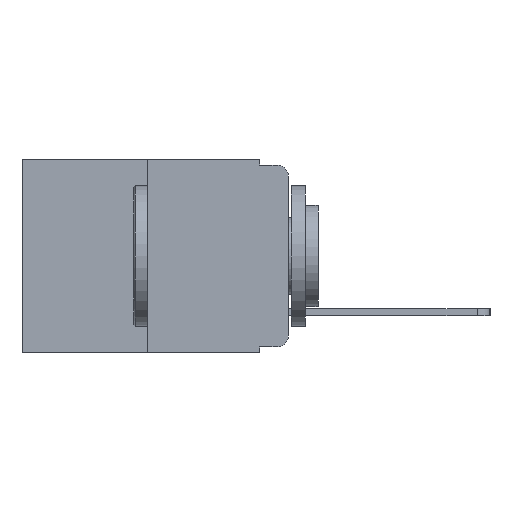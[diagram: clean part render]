
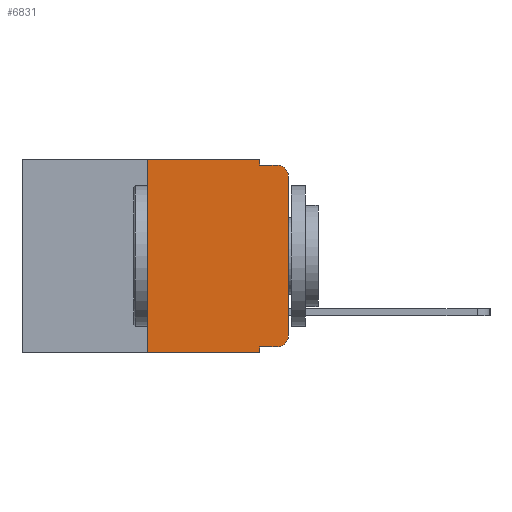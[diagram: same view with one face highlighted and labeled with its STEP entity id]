
A CAD part, left-side view. The second image highlights one B-rep face of the part: STEP entity #6831.
In plain terms, the highlighted planar face has unit normal (-1, 0, 0).
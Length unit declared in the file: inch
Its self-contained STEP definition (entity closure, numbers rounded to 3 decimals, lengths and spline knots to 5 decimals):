
#85 = EDGE_CURVE ( 'NONE', #959, #15943, #3698, .T. ) ;
#376 = EDGE_CURVE ( 'NONE', #1472, #6557, #10152, .T. ) ;
#380 = EDGE_CURVE ( 'NONE', #6557, #20384, #722, .T. ) ;
#412 = EDGE_CURVE ( 'NONE', #9446, #20384, #13553, .T. ) ;
#414 = EDGE_CURVE ( 'NONE', #8505, #9446, #9124, .T. ) ;
#418 = EDGE_CURVE ( 'NONE', #959, #8233, #17444, .T. ) ;
#449 = EDGE_CURVE ( 'NONE', #7345, #15943, #2830, .T. ) ;
#456 = EDGE_CURVE ( 'NONE', #7345, #13118, #6999, .T. ) ;
#485 = EDGE_CURVE ( 'NONE', #13118, #1472, #1667, .T. ) ;
#707 = ORIENTED_EDGE ( 'NONE', *, *, #85, .T. ) ;
#722 = CIRCLE ( 'NONE', #8372, 0.02 ) ;
#959 = VERTEX_POINT ( 'NONE', #21554 ) ;
#1197 = DIRECTION ( 'NONE',  ( 0., -1., 0. ) ) ;
#1244 = DIRECTION ( 'NONE',  ( 0., -1., 0. ) ) ;
#1324 = ORIENTED_EDGE ( 'NONE', *, *, #380, .T. ) ;
#1472 = VERTEX_POINT ( 'NONE', #10882 ) ;
#1580 = CARTESIAN_POINT ( 'NONE',  ( 0., 0.02, -0.313 ) ) ;
#1667 = CIRCLE ( 'NONE', #4444, 0.02 ) ;
#1971 = ORIENTED_EDGE ( 'NONE', *, *, #456, .T. ) ;
#2003 = DIRECTION ( 'NONE',  ( -1., 0., 0. ) ) ;
#2273 = VECTOR ( 'NONE', #15319, 39.37008 ) ;
#2487 = CARTESIAN_POINT ( 'NONE',  ( 0., 0.051, 0. ) ) ;
#2830 = LINE ( 'NONE', #19865, #12493 ) ;
#3638 = ORIENTED_EDGE ( 'NONE', *, *, #414, .F. ) ;
#3698 = LINE ( 'NONE', #3731, #15667 ) ;
#3731 = CARTESIAN_POINT ( 'NONE',  ( 0., 0.473, -0.343 ) ) ;
#4444 = AXIS2_PLACEMENT_3D ( 'NONE', #1580, #14850, #15850 ) ;
#4504 = ORIENTED_EDGE ( 'NONE', *, *, #8119, .F. ) ;
#6193 = ORIENTED_EDGE ( 'NONE', *, *, #449, .F. ) ;
#6557 = VERTEX_POINT ( 'NONE', #20233 ) ;
#6738 = ORIENTED_EDGE ( 'NONE', *, *, #485, .T. ) ;
#6809 = CARTESIAN_POINT ( 'NONE',  ( 0., 0.051, -0.01 ) ) ;
#6831 = ADVANCED_FACE ( 'NONE', ( #8247 ), #16004, .F. ) ;
#6999 = LINE ( 'NONE', #7758, #2273 ) ;
#7345 = VERTEX_POINT ( 'NONE', #9609 ) ;
#7408 = EDGE_LOOP ( 'NONE', ( #20463, #1324, #19471, #3638, #4504, #14064, #707, #6193, #1971, #6738 ) ) ;
#7517 = CARTESIAN_POINT ( 'NONE',  ( 0., 0.051, -0.01 ) ) ;
#7758 = CARTESIAN_POINT ( 'NONE',  ( 0., 0.051, -0.333 ) ) ;
#8119 = EDGE_CURVE ( 'NONE', #8233, #8505, #14284, .T. ) ;
#8233 = VERTEX_POINT ( 'NONE', #10360 ) ;
#8247 = FACE_OUTER_BOUND ( 'NONE', #7408, .T. ) ;
#8372 = AXIS2_PLACEMENT_3D ( 'NONE', #18303, #2003, #18585 ) ;
#8505 = VERTEX_POINT ( 'NONE', #2487 ) ;
#8602 = VECTOR ( 'NONE', #14365, 39.37008 ) ;
#9100 = DIRECTION ( 'NONE',  ( 0., 0., -1. ) ) ;
#9113 = CARTESIAN_POINT ( 'NONE',  ( 0., 0.051, 0. ) ) ;
#9124 = LINE ( 'NONE', #9113, #14076 ) ;
#9446 = VERTEX_POINT ( 'NONE', #6809 ) ;
#9609 = CARTESIAN_POINT ( 'NONE',  ( 0., 0.051, -0.333 ) ) ;
#10152 = LINE ( 'NONE', #13634, #18480 ) ;
#10360 = CARTESIAN_POINT ( 'NONE',  ( 0., 0.25, 0. ) ) ;
#10882 = CARTESIAN_POINT ( 'NONE',  ( 0., 0., -0.313 ) ) ;
#11143 = AXIS2_PLACEMENT_3D ( 'NONE', #19725, #21334, #11439 ) ;
#11439 = DIRECTION ( 'NONE',  ( 0., 0., -1. ) ) ;
#11524 = CARTESIAN_POINT ( 'NONE',  ( 0., 0.25, 0. ) ) ;
#12154 = VECTOR ( 'NONE', #1244, 39.37008 ) ;
#12493 = VECTOR ( 'NONE', #19282, 39.37008 ) ;
#13020 = DIRECTION ( 'NONE',  ( 0., 0., 1. ) ) ;
#13118 = VERTEX_POINT ( 'NONE', #15494 ) ;
#13553 = LINE ( 'NONE', #7517, #21765 ) ;
#13634 = CARTESIAN_POINT ( 'NONE',  ( 0., 0., 0. ) ) ;
#14064 = ORIENTED_EDGE ( 'NONE', *, *, #418, .F. ) ;
#14076 = VECTOR ( 'NONE', #9100, 39.37008 ) ;
#14284 = LINE ( 'NONE', #15079, #12154 ) ;
#14365 = DIRECTION ( 'NONE',  ( 0., 0., 1. ) ) ;
#14850 = DIRECTION ( 'NONE',  ( -1., 0., 0. ) ) ;
#15079 = CARTESIAN_POINT ( 'NONE',  ( 0., 0.473, 0. ) ) ;
#15319 = DIRECTION ( 'NONE',  ( 0., -1., 0. ) ) ;
#15494 = CARTESIAN_POINT ( 'NONE',  ( 0., 0.02, -0.333 ) ) ;
#15667 = VECTOR ( 'NONE', #18760, 39.37008 ) ;
#15850 = DIRECTION ( 'NONE',  ( 0., 0., -1. ) ) ;
#15943 = VERTEX_POINT ( 'NONE', #19758 ) ;
#16004 = PLANE ( 'NONE',  #11143 ) ;
#16786 = CARTESIAN_POINT ( 'NONE',  ( 0., 0.02, -0.01 ) ) ;
#17444 = LINE ( 'NONE', #11524, #8602 ) ;
#18303 = CARTESIAN_POINT ( 'NONE',  ( 0., 0.02, -0.03 ) ) ;
#18480 = VECTOR ( 'NONE', #13020, 39.37008 ) ;
#18585 = DIRECTION ( 'NONE',  ( 0., 0., -1. ) ) ;
#18760 = DIRECTION ( 'NONE',  ( 0., -1., 0. ) ) ;
#19282 = DIRECTION ( 'NONE',  ( 0., 0., -1. ) ) ;
#19471 = ORIENTED_EDGE ( 'NONE', *, *, #412, .F. ) ;
#19725 = CARTESIAN_POINT ( 'NONE',  ( 0., 0.473, 0. ) ) ;
#19758 = CARTESIAN_POINT ( 'NONE',  ( 0., 0.051, -0.343 ) ) ;
#19865 = CARTESIAN_POINT ( 'NONE',  ( 0., 0.051, 0. ) ) ;
#20233 = CARTESIAN_POINT ( 'NONE',  ( 0., 0., -0.03 ) ) ;
#20384 = VERTEX_POINT ( 'NONE', #16786 ) ;
#20463 = ORIENTED_EDGE ( 'NONE', *, *, #376, .T. ) ;
#21334 = DIRECTION ( 'NONE',  ( 1., 0., 0. ) ) ;
#21554 = CARTESIAN_POINT ( 'NONE',  ( 0., 0.25, -0.343 ) ) ;
#21765 = VECTOR ( 'NONE', #1197, 39.37008 ) ;
